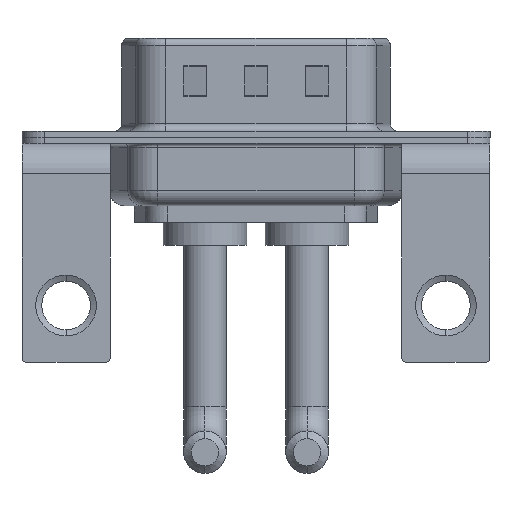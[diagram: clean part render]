
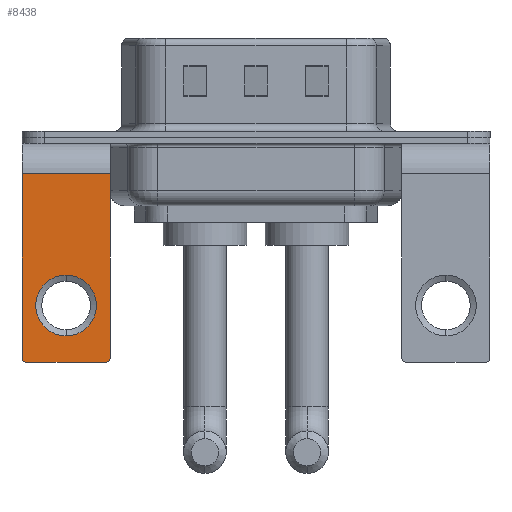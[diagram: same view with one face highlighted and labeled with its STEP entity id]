
A CAD part, front view. The second image highlights one B-rep face of the part: STEP entity #8438.
In plain terms, the highlighted planar face has unit normal (0, -1, 0).
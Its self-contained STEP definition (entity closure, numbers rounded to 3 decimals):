
#404 = EDGE_LOOP ( 'NONE', ( #4445, #690 ) ) ;
#414 = EDGE_LOOP ( 'NONE', ( #11814, #6102, #12427, #1231, #10253, #8425 ) ) ;
#690 = ORIENTED_EDGE ( 'NONE', *, *, #13844, .T. ) ;
#1000 = CARTESIAN_POINT ( 'NONE',  ( 2.9, -6.25, -2.4 ) ) ;
#1034 = VERTEX_POINT ( 'NONE', #6794 ) ;
#1115 = DIRECTION ( 'NONE',  ( 0., -1., 0. ) ) ;
#1164 = FACE_BOUND ( 'NONE', #404, .T. ) ;
#1231 = ORIENTED_EDGE ( 'NONE', *, *, #14217, .T. ) ;
#1233 = DIRECTION ( 'NONE',  ( 0., 1., 0. ) ) ;
#1547 = DIRECTION ( 'NONE',  ( 0., 0., 1. ) ) ;
#1571 = CARTESIAN_POINT ( 'NONE',  ( -2.9, -6.25, -14.55 ) ) ;
#1577 = LINE ( 'NONE', #5309, #11690 ) ;
#1767 = VERTEX_POINT ( 'NONE', #1571 ) ;
#1822 = VERTEX_POINT ( 'NONE', #5304 ) ;
#2766 = AXIS2_PLACEMENT_3D ( 'NONE', #3585, #3509, #10689 ) ;
#3186 = EDGE_CURVE ( 'NONE', #11209, #6569, #4260, .T. ) ;
#3258 = CARTESIAN_POINT ( 'NONE',  ( -2.65, -6.25, -14.8 ) ) ;
#3368 = VECTOR ( 'NONE', #12543, 1000. ) ;
#3509 = DIRECTION ( 'NONE',  ( 0., 1., 0. ) ) ;
#3585 = CARTESIAN_POINT ( 'NONE',  ( 0., -6.25, -11.07 ) ) ;
#3625 = VECTOR ( 'NONE', #6958, 1000. ) ;
#3725 = CARTESIAN_POINT ( 'NONE',  ( 2.9, -6.25, -2.4 ) ) ;
#4260 = CIRCLE ( 'NONE', #2766, 2. ) ;
#4281 = EDGE_CURVE ( 'NONE', #7045, #1767, #6253, .T. ) ;
#4445 = ORIENTED_EDGE ( 'NONE', *, *, #3186, .T. ) ;
#4503 = DIRECTION ( 'NONE',  ( 0., 0., 1. ) ) ;
#4537 = CARTESIAN_POINT ( 'NONE',  ( 2.65, -6.25, -14.8 ) ) ;
#4851 = CIRCLE ( 'NONE', #8296, 0.25 ) ;
#5304 = CARTESIAN_POINT ( 'NONE',  ( 2.9, -6.25, -2.4 ) ) ;
#5309 = CARTESIAN_POINT ( 'NONE',  ( 2.9, -6.25, -2.4 ) ) ;
#5531 = EDGE_CURVE ( 'NONE', #9393, #12126, #6610, .T. ) ;
#6102 = ORIENTED_EDGE ( 'NONE', *, *, #9456, .T. ) ;
#6253 = LINE ( 'NONE', #6328, #12787 ) ;
#6328 = CARTESIAN_POINT ( 'NONE',  ( -2.9, -6.25, -2.4 ) ) ;
#6569 = VERTEX_POINT ( 'NONE', #8005 ) ;
#6610 = LINE ( 'NONE', #7525, #3368 ) ;
#6794 = CARTESIAN_POINT ( 'NONE',  ( 2.9, -6.25, -14.55 ) ) ;
#6889 = LINE ( 'NONE', #1000, #3625 ) ;
#6958 = DIRECTION ( 'NONE',  ( -1., 0., 0. ) ) ;
#7045 = VERTEX_POINT ( 'NONE', #13289 ) ;
#7318 = CARTESIAN_POINT ( 'NONE',  ( -2.65, -6.25, -14.55 ) ) ;
#7432 = EDGE_CURVE ( 'NONE', #1822, #1034, #1577, .T. ) ;
#7525 = CARTESIAN_POINT ( 'NONE',  ( 2.9, -6.25, -14.8 ) ) ;
#8005 = CARTESIAN_POINT ( 'NONE',  ( 0., -6.25, -9.07 ) ) ;
#8201 = CARTESIAN_POINT ( 'NONE',  ( 2.65, -6.25, -14.55 ) ) ;
#8296 = AXIS2_PLACEMENT_3D ( 'NONE', #7318, #1115, #12934 ) ;
#8425 = ORIENTED_EDGE ( 'NONE', *, *, #9801, .T. ) ;
#8438 = ADVANCED_FACE ( 'NONE', ( #1164, #10675 ), #14368, .F. ) ;
#9393 = VERTEX_POINT ( 'NONE', #4537 ) ;
#9456 = EDGE_CURVE ( 'NONE', #1767, #12126, #4851, .T. ) ;
#9751 = AXIS2_PLACEMENT_3D ( 'NONE', #3725, #1233, #13283 ) ;
#9768 = AXIS2_PLACEMENT_3D ( 'NONE', #8201, #15080, #4503 ) ;
#9801 = EDGE_CURVE ( 'NONE', #1822, #7045, #6889, .T. ) ;
#10253 = ORIENTED_EDGE ( 'NONE', *, *, #7432, .F. ) ;
#10254 = AXIS2_PLACEMENT_3D ( 'NONE', #15253, #12071, #1547 ) ;
#10675 = FACE_OUTER_BOUND ( 'NONE', #414, .T. ) ;
#10689 = DIRECTION ( 'NONE',  ( 0., 0., 1. ) ) ;
#11039 = DIRECTION ( 'NONE',  ( 0., 0., -1. ) ) ;
#11209 = VERTEX_POINT ( 'NONE', #12504 ) ;
#11690 = VECTOR ( 'NONE', #12398, 1000. ) ;
#11722 = CIRCLE ( 'NONE', #10254, 2. ) ;
#11814 = ORIENTED_EDGE ( 'NONE', *, *, #4281, .T. ) ;
#12071 = DIRECTION ( 'NONE',  ( 0., 1., 0. ) ) ;
#12126 = VERTEX_POINT ( 'NONE', #3258 ) ;
#12398 = DIRECTION ( 'NONE',  ( 0., 0., -1. ) ) ;
#12427 = ORIENTED_EDGE ( 'NONE', *, *, #5531, .F. ) ;
#12504 = CARTESIAN_POINT ( 'NONE',  ( 0., -6.25, -13.07 ) ) ;
#12543 = DIRECTION ( 'NONE',  ( -1., 0., 0. ) ) ;
#12787 = VECTOR ( 'NONE', #11039, 1000. ) ;
#12934 = DIRECTION ( 'NONE',  ( 0., 0., 1. ) ) ;
#13283 = DIRECTION ( 'NONE',  ( 0., 0., 1. ) ) ;
#13289 = CARTESIAN_POINT ( 'NONE',  ( -2.9, -6.25, -2.4 ) ) ;
#13712 = CIRCLE ( 'NONE', #9768, 0.25 ) ;
#13844 = EDGE_CURVE ( 'NONE', #6569, #11209, #11722, .T. ) ;
#14217 = EDGE_CURVE ( 'NONE', #9393, #1034, #13712, .T. ) ;
#14368 = PLANE ( 'NONE',  #9751 ) ;
#15080 = DIRECTION ( 'NONE',  ( 0., -1., 0. ) ) ;
#15253 = CARTESIAN_POINT ( 'NONE',  ( 0., -6.25, -11.07 ) ) ;
